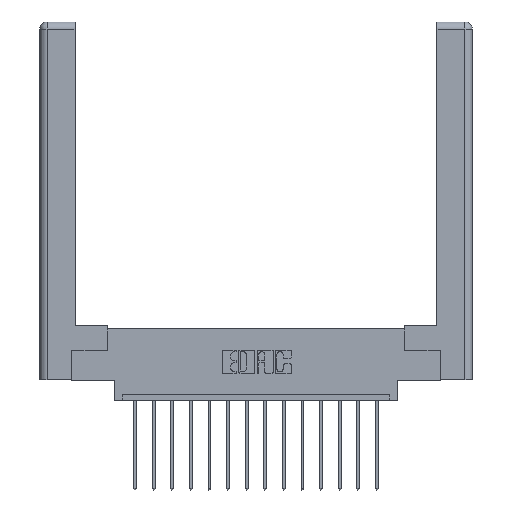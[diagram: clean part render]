
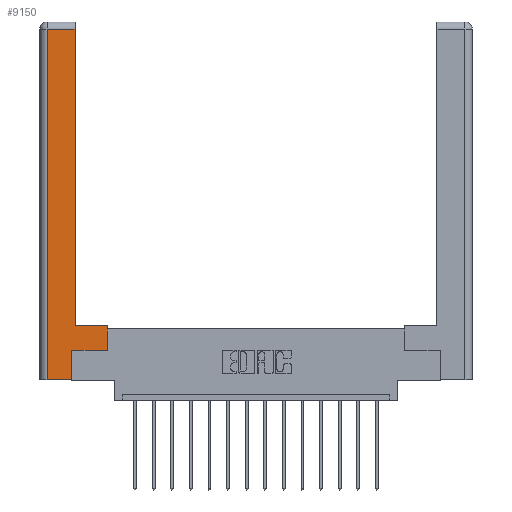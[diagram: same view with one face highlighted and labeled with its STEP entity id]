
A CAD part, top view. The second image highlights one B-rep face of the part: STEP entity #9150.
In plain terms, the highlighted planar face has unit normal (0, 0, 1).
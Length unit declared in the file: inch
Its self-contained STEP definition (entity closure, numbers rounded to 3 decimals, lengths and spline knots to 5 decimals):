
#328 = DIRECTION ( 'NONE',  ( 0., 1., 0. ) ) ;
#493 = EDGE_CURVE ( 'NONE', #14964, #13861, #15952, .T. ) ;
#595 = CARTESIAN_POINT ( 'NONE',  ( 0.565, 0.245, 0. ) ) ;
#807 = CARTESIAN_POINT ( 'NONE',  ( 0.565, 0.45, 0. ) ) ;
#1232 = PLANE ( 'NONE',  #10397 ) ;
#1339 = DIRECTION ( 'NONE',  ( 0., 0., -1. ) ) ;
#2502 = CARTESIAN_POINT ( 'NONE',  ( 0.0615, 0., 0. ) ) ;
#2730 = LINE ( 'NONE', #10280, #9215 ) ;
#2902 = CARTESIAN_POINT ( 'NONE',  ( 0.565, 0.45, 0. ) ) ;
#3773 = LINE ( 'NONE', #6738, #11099 ) ;
#3809 = DIRECTION ( 'NONE',  ( -1., 0., 0. ) ) ;
#4086 = ORIENTED_EDGE ( 'NONE', *, *, #12997, .T. ) ;
#4726 = VECTOR ( 'NONE', #12737, 39.37008 ) ;
#4796 = VERTEX_POINT ( 'NONE', #6987 ) ;
#4802 = VECTOR ( 'NONE', #5126, 39.37008 ) ;
#4900 = CARTESIAN_POINT ( 'NONE',  ( 0.0615, 2.94, 0. ) ) ;
#4903 = EDGE_LOOP ( 'NONE', ( #5464, #14080, #10413, #10718, #11577, #12282, #4086, #9331 ) ) ;
#5126 = DIRECTION ( 'NONE',  ( -1., 0., 0. ) ) ;
#5299 = VERTEX_POINT ( 'NONE', #10518 ) ;
#5464 = ORIENTED_EDGE ( 'NONE', *, *, #12747, .T. ) ;
#6169 = LINE ( 'NONE', #10749, #11447 ) ;
#6388 = CARTESIAN_POINT ( 'NONE',  ( 0.295, 0.45, 0. ) ) ;
#6583 = CARTESIAN_POINT ( 'NONE',  ( 0.295, 0.45, 0. ) ) ;
#6738 = CARTESIAN_POINT ( 'NONE',  ( 0.265, 0.245, 0. ) ) ;
#6842 = DIRECTION ( 'NONE',  ( 0., 1., 0. ) ) ;
#6987 = CARTESIAN_POINT ( 'NONE',  ( 0.0615, 0., 0. ) ) ;
#7192 = CARTESIAN_POINT ( 'NONE',  ( 0.265, 0., 0. ) ) ;
#7462 = EDGE_CURVE ( 'NONE', #11513, #8890, #11908, .T. ) ;
#7976 = VECTOR ( 'NONE', #12565, 39.37008 ) ;
#8057 = VECTOR ( 'NONE', #15321, 39.37008 ) ;
#8650 = CARTESIAN_POINT ( 'NONE',  ( 0.565, 0.245, 0. ) ) ;
#8779 = LINE ( 'NONE', #595, #9040 ) ;
#8890 = VERTEX_POINT ( 'NONE', #6583 ) ;
#8902 = CARTESIAN_POINT ( 'NONE',  ( 0., 0., 0. ) ) ;
#9040 = VECTOR ( 'NONE', #9988, 39.37008 ) ;
#9113 = EDGE_CURVE ( 'NONE', #4796, #12474, #2730, .T. ) ;
#9150 = ADVANCED_FACE ( 'NONE', ( #13053 ), #1232, .F. ) ;
#9215 = VECTOR ( 'NONE', #12944, 39.37008 ) ;
#9331 = ORIENTED_EDGE ( 'NONE', *, *, #7462, .T. ) ;
#9506 = VERTEX_POINT ( 'NONE', #8650 ) ;
#9988 = DIRECTION ( 'NONE',  ( 1., 0., 0. ) ) ;
#10280 = CARTESIAN_POINT ( 'NONE',  ( 0.265, 0., 0. ) ) ;
#10397 = AXIS2_PLACEMENT_3D ( 'NONE', #8902, #1339, #3809 ) ;
#10412 = CARTESIAN_POINT ( 'NONE',  ( 0.295, 2.94, 0. ) ) ;
#10413 = ORIENTED_EDGE ( 'NONE', *, *, #12577, .T. ) ;
#10518 = CARTESIAN_POINT ( 'NONE',  ( 0.265, 0.245, 0. ) ) ;
#10718 = ORIENTED_EDGE ( 'NONE', *, *, #9113, .T. ) ;
#10749 = CARTESIAN_POINT ( 'NONE',  ( 0.295, 3., 0. ) ) ;
#11099 = VECTOR ( 'NONE', #328, 39.37008 ) ;
#11447 = VECTOR ( 'NONE', #6842, 39.37008 ) ;
#11513 = VERTEX_POINT ( 'NONE', #2902 ) ;
#11577 = ORIENTED_EDGE ( 'NONE', *, *, #16716, .T. ) ;
#11908 = LINE ( 'NONE', #6388, #4802 ) ;
#12282 = ORIENTED_EDGE ( 'NONE', *, *, #14270, .T. ) ;
#12474 = VERTEX_POINT ( 'NONE', #7192 ) ;
#12565 = DIRECTION ( 'NONE',  ( 0., 1., 0. ) ) ;
#12577 = EDGE_CURVE ( 'NONE', #13861, #4796, #13047, .T. ) ;
#12737 = DIRECTION ( 'NONE',  ( 0., -1., 0. ) ) ;
#12747 = EDGE_CURVE ( 'NONE', #8890, #14964, #6169, .T. ) ;
#12827 = LINE ( 'NONE', #807, #7976 ) ;
#12944 = DIRECTION ( 'NONE',  ( 1., 0., 0. ) ) ;
#12997 = EDGE_CURVE ( 'NONE', #9506, #11513, #12827, .T. ) ;
#13047 = LINE ( 'NONE', #2502, #4726 ) ;
#13053 = FACE_OUTER_BOUND ( 'NONE', #4903, .T. ) ;
#13861 = VERTEX_POINT ( 'NONE', #4900 ) ;
#14080 = ORIENTED_EDGE ( 'NONE', *, *, #493, .T. ) ;
#14270 = EDGE_CURVE ( 'NONE', #5299, #9506, #8779, .T. ) ;
#14964 = VERTEX_POINT ( 'NONE', #10412 ) ;
#15321 = DIRECTION ( 'NONE',  ( -1., 0., 0. ) ) ;
#15952 = LINE ( 'NONE', #16426, #8057 ) ;
#16426 = CARTESIAN_POINT ( 'NONE',  ( 0.0615, 2.94, 0. ) ) ;
#16716 = EDGE_CURVE ( 'NONE', #12474, #5299, #3773, .T. ) ;
